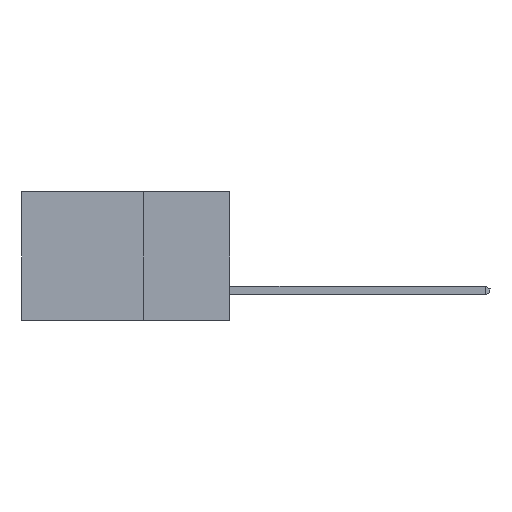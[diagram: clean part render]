
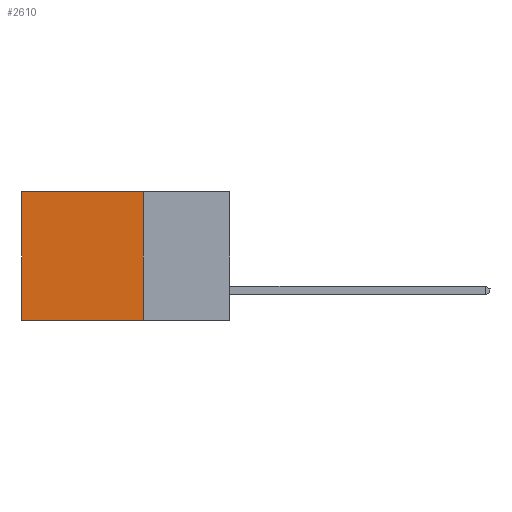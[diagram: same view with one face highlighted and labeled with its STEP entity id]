
A CAD part, left-side view. The second image highlights one B-rep face of the part: STEP entity #2610.
In plain terms, the highlighted planar face has unit normal (-1, 0, 0).
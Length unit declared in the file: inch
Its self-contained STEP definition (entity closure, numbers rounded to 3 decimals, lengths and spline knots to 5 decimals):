
#466 = VECTOR ( 'NONE', #7182, 39.37008 ) ;
#1138 = LINE ( 'NONE', #25213, #466 ) ;
#1265 = DIRECTION ( 'NONE',  ( 0., 1., 0. ) ) ;
#1754 = ORIENTED_EDGE ( 'NONE', *, *, #17843, .F. ) ;
#2420 = CARTESIAN_POINT ( 'NONE',  ( 0.2615, 0.25, 0. ) ) ;
#2610 = ADVANCED_FACE ( 'NONE', ( #7004 ), #8586, .F. ) ;
#2636 = VERTEX_POINT ( 'NONE', #17116 ) ;
#3586 = EDGE_CURVE ( 'NONE', #25312, #2636, #17539, .T. ) ;
#3626 = EDGE_CURVE ( 'NONE', #2636, #17646, #9425, .T. ) ;
#5781 = LINE ( 'NONE', #20125, #6775 ) ;
#6775 = VECTOR ( 'NONE', #8155, 39.37008 ) ;
#7004 = FACE_OUTER_BOUND ( 'NONE', #21580, .T. ) ;
#7182 = DIRECTION ( 'NONE',  ( 0., 1., 0. ) ) ;
#8155 = DIRECTION ( 'NONE',  ( 0., 0., -1. ) ) ;
#8586 = PLANE ( 'NONE',  #13367 ) ;
#8950 = VERTEX_POINT ( 'NONE', #24173 ) ;
#9425 = LINE ( 'NONE', #13625, #18868 ) ;
#9818 = CARTESIAN_POINT ( 'NONE',  ( 0.2615, 0.25, 0. ) ) ;
#11277 = ORIENTED_EDGE ( 'NONE', *, *, #16798, .F. ) ;
#12151 = VECTOR ( 'NONE', #1265, 39.37008 ) ;
#13367 = AXIS2_PLACEMENT_3D ( 'NONE', #14635, #22684, #20974 ) ;
#13625 = CARTESIAN_POINT ( 'NONE',  ( 0.2615, 0.6, -0.37 ) ) ;
#14635 = CARTESIAN_POINT ( 'NONE',  ( 0.2615, 0.25, -0.37 ) ) ;
#16798 = EDGE_CURVE ( 'NONE', #8950, #17646, #1138, .T. ) ;
#17116 = CARTESIAN_POINT ( 'NONE',  ( 0.2615, 0.6, 0. ) ) ;
#17380 = ORIENTED_EDGE ( 'NONE', *, *, #3586, .T. ) ;
#17539 = LINE ( 'NONE', #9818, #12151 ) ;
#17646 = VERTEX_POINT ( 'NONE', #22790 ) ;
#17843 = EDGE_CURVE ( 'NONE', #25312, #8950, #5781, .T. ) ;
#18868 = VECTOR ( 'NONE', #25462, 39.37008 ) ;
#20125 = CARTESIAN_POINT ( 'NONE',  ( 0.2615, 0.25, -0.37 ) ) ;
#20852 = ORIENTED_EDGE ( 'NONE', *, *, #3626, .T. ) ;
#20974 = DIRECTION ( 'NONE',  ( 0., 0., -1. ) ) ;
#21580 = EDGE_LOOP ( 'NONE', ( #20852, #11277, #1754, #17380 ) ) ;
#22684 = DIRECTION ( 'NONE',  ( 1., 0., 0. ) ) ;
#22790 = CARTESIAN_POINT ( 'NONE',  ( 0.2615, 0.6, -0.37 ) ) ;
#24173 = CARTESIAN_POINT ( 'NONE',  ( 0.2615, 0.25, -0.37 ) ) ;
#25213 = CARTESIAN_POINT ( 'NONE',  ( 0.2615, 0.25, -0.37 ) ) ;
#25312 = VERTEX_POINT ( 'NONE', #2420 ) ;
#25462 = DIRECTION ( 'NONE',  ( 0., 0., -1. ) ) ;
